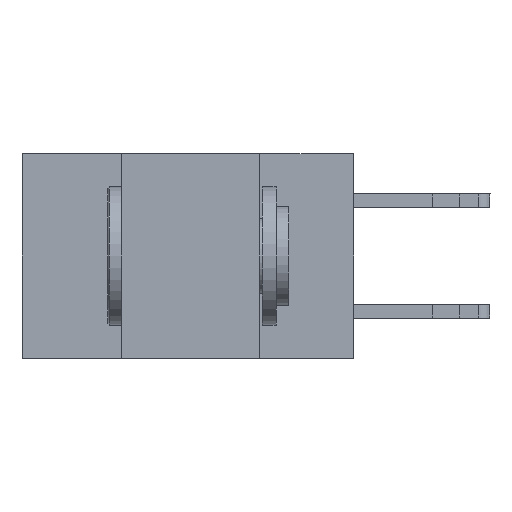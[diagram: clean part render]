
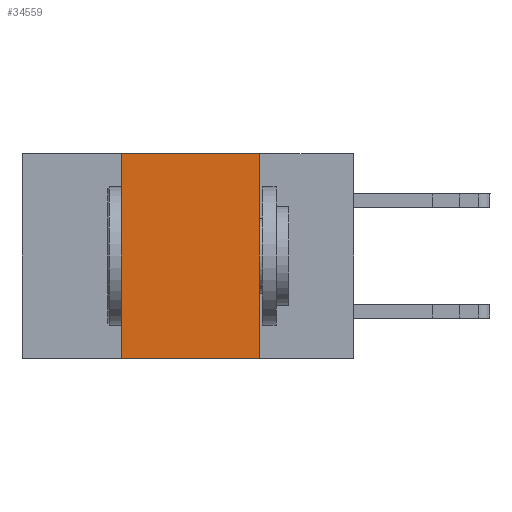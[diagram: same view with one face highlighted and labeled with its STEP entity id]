
A CAD part, left-side view. The second image highlights one B-rep face of the part: STEP entity #34559.
In plain terms, the highlighted planar face has unit normal (-1, 0, 0).
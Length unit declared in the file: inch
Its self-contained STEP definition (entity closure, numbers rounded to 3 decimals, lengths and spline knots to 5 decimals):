
#175 = AXIS2_PLACEMENT_3D ( 'NONE', #9782, #22045, #16367 ) ;
#854 = CARTESIAN_POINT ( 'NONE',  ( 0., 0.6, -0.37 ) ) ;
#934 = EDGE_CURVE ( 'NONE', #28938, #5925, #11052, .T. ) ;
#2066 = ORIENTED_EDGE ( 'NONE', *, *, #15875, .T. ) ;
#3761 = DIRECTION ( 'NONE',  ( 0., -1., 0. ) ) ;
#5925 = VERTEX_POINT ( 'NONE', #15436 ) ;
#6370 = CARTESIAN_POINT ( 'NONE',  ( 0., 0.17, 0. ) ) ;
#7002 = VERTEX_POINT ( 'NONE', #6370 ) ;
#8865 = CARTESIAN_POINT ( 'NONE',  ( 0., 0.42, 0. ) ) ;
#9079 = VECTOR ( 'NONE', #3761, 39.37008 ) ;
#9386 = FACE_OUTER_BOUND ( 'NONE', #16739, .T. ) ;
#9782 = CARTESIAN_POINT ( 'NONE',  ( 0., 0.6, 0. ) ) ;
#11052 = LINE ( 'NONE', #8865, #29698 ) ;
#12615 = LINE ( 'NONE', #14144, #15282 ) ;
#12904 = EDGE_CURVE ( 'NONE', #7002, #13828, #12615, .T. ) ;
#13557 = DIRECTION ( 'NONE',  ( 0., -1., 0. ) ) ;
#13828 = VERTEX_POINT ( 'NONE', #18252 ) ;
#14144 = CARTESIAN_POINT ( 'NONE',  ( 0., 0.17, 0. ) ) ;
#15282 = VECTOR ( 'NONE', #16984, 39.37008 ) ;
#15436 = CARTESIAN_POINT ( 'NONE',  ( 0., 0.42, 0. ) ) ;
#15875 = EDGE_CURVE ( 'NONE', #28938, #13828, #29979, .T. ) ;
#16367 = DIRECTION ( 'NONE',  ( 0., 0., -1. ) ) ;
#16739 = EDGE_LOOP ( 'NONE', ( #16845, #26738, #26580, #2066 ) ) ;
#16845 = ORIENTED_EDGE ( 'NONE', *, *, #12904, .F. ) ;
#16984 = DIRECTION ( 'NONE',  ( 0., 0., -1. ) ) ;
#17235 = EDGE_CURVE ( 'NONE', #5925, #7002, #28970, .T. ) ;
#18252 = CARTESIAN_POINT ( 'NONE',  ( 0., 0.17, -0.37 ) ) ;
#19109 = CARTESIAN_POINT ( 'NONE',  ( 0., 0.6, 0. ) ) ;
#20117 = DIRECTION ( 'NONE',  ( 0., 0., 1. ) ) ;
#22045 = DIRECTION ( 'NONE',  ( 1., 0., 0. ) ) ;
#24043 = CARTESIAN_POINT ( 'NONE',  ( 0., 0.42, -0.37 ) ) ;
#26580 = ORIENTED_EDGE ( 'NONE', *, *, #934, .F. ) ;
#26738 = ORIENTED_EDGE ( 'NONE', *, *, #17235, .F. ) ;
#26753 = PLANE ( 'NONE',  #175 ) ;
#28938 = VERTEX_POINT ( 'NONE', #24043 ) ;
#28970 = LINE ( 'NONE', #19109, #31701 ) ;
#29698 = VECTOR ( 'NONE', #20117, 39.37008 ) ;
#29979 = LINE ( 'NONE', #854, #9079 ) ;
#31701 = VECTOR ( 'NONE', #13557, 39.37008 ) ;
#34559 = ADVANCED_FACE ( 'NONE', ( #9386 ), #26753, .F. ) ;
